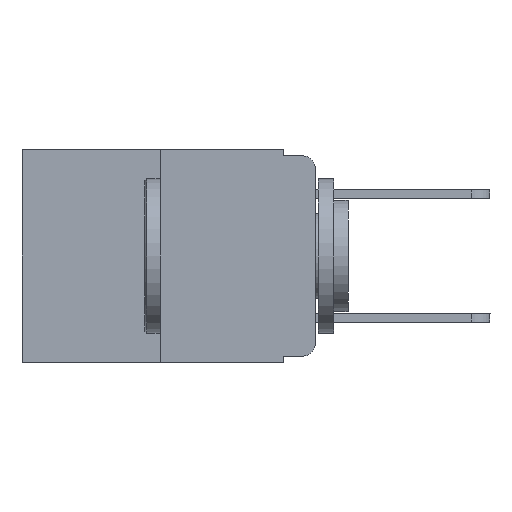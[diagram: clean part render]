
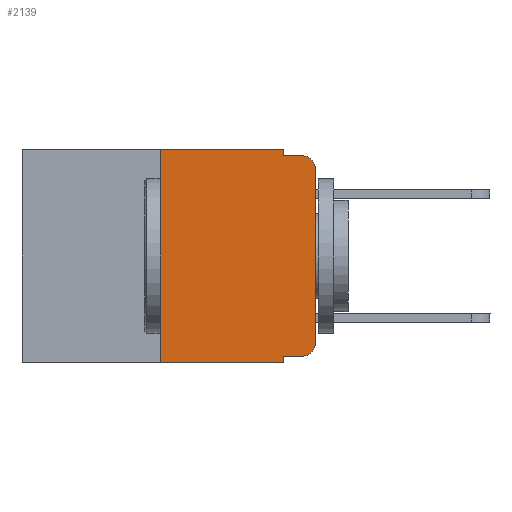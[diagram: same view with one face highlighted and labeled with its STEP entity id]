
A CAD part, left-side view. The second image highlights one B-rep face of the part: STEP entity #2139.
In plain terms, the highlighted planar face has unit normal (-1, 0, 0).
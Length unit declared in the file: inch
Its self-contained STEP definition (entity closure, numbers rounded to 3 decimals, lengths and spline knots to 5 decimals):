
#105 = ORIENTED_EDGE ( 'NONE', *, *, #9672, .T. ) ;
#133 = VERTEX_POINT ( 'NONE', #2165 ) ;
#196 = ORIENTED_EDGE ( 'NONE', *, *, #19127, .T. ) ;
#374 = DIRECTION ( 'NONE',  ( 0., -1., 0. ) ) ;
#551 = CARTESIAN_POINT ( 'NONE',  ( 0., 0.02, -0.333 ) ) ;
#833 = DIRECTION ( 'NONE',  ( 0., -1., 0. ) ) ;
#955 = VECTOR ( 'NONE', #6826, 39.37008 ) ;
#981 = ORIENTED_EDGE ( 'NONE', *, *, #5267, .F. ) ;
#1406 = VECTOR ( 'NONE', #11845, 39.37008 ) ;
#1689 = VECTOR ( 'NONE', #833, 39.37008 ) ;
#2076 = EDGE_CURVE ( 'NONE', #12194, #8898, #11866, .T. ) ;
#2139 = ADVANCED_FACE ( 'NONE', ( #11354 ), #15346, .F. ) ;
#2165 = CARTESIAN_POINT ( 'NONE',  ( 0., 0.02, -0.01 ) ) ;
#2209 = EDGE_CURVE ( 'NONE', #13697, #2356, #12379, .T. ) ;
#2356 = VERTEX_POINT ( 'NONE', #6018 ) ;
#2637 = CARTESIAN_POINT ( 'NONE',  ( 0., 0.25, 0. ) ) ;
#2941 = ORIENTED_EDGE ( 'NONE', *, *, #13623, .T. ) ;
#3417 = CARTESIAN_POINT ( 'NONE',  ( 0., 0.051, -0.01 ) ) ;
#3504 = DIRECTION ( 'NONE',  ( 0., 0., 1. ) ) ;
#3526 = CARTESIAN_POINT ( 'NONE',  ( 0., 0.051, 0. ) ) ;
#3606 = DIRECTION ( 'NONE',  ( 1., 0., 0. ) ) ;
#3746 = CARTESIAN_POINT ( 'NONE',  ( 0., 0.473, 0. ) ) ;
#3792 = ORIENTED_EDGE ( 'NONE', *, *, #3829, .F. ) ;
#3829 = EDGE_CURVE ( 'NONE', #18130, #133, #15954, .T. ) ;
#4917 = LINE ( 'NONE', #19676, #15035 ) ;
#5001 = VECTOR ( 'NONE', #3504, 39.37008 ) ;
#5251 = DIRECTION ( 'NONE',  ( 0., 0., -1. ) ) ;
#5267 = EDGE_CURVE ( 'NONE', #15118, #12194, #14366, .T. ) ;
#5407 = EDGE_LOOP ( 'NONE', ( #14803, #196, #3792, #10433, #10641, #981, #105, #11009, #20525, #2941 ) ) ;
#5794 = DIRECTION ( 'NONE',  ( -1., 0., 0. ) ) ;
#6018 = CARTESIAN_POINT ( 'NONE',  ( 0., 0., -0.03 ) ) ;
#6826 = DIRECTION ( 'NONE',  ( 0., -1., 0. ) ) ;
#7186 = EDGE_CURVE ( 'NONE', #13877, #10578, #13837, .T. ) ;
#7268 = EDGE_CURVE ( 'NONE', #13877, #12577, #12021, .T. ) ;
#7383 = DIRECTION ( 'NONE',  ( 0., 0., 1. ) ) ;
#7666 = CARTESIAN_POINT ( 'NONE',  ( 0., 0.051, 0. ) ) ;
#7942 = VECTOR ( 'NONE', #7383, 39.37008 ) ;
#8195 = CARTESIAN_POINT ( 'NONE',  ( 0., 0., -0.313 ) ) ;
#8267 = CARTESIAN_POINT ( 'NONE',  ( 0., 0.02, -0.313 ) ) ;
#8898 = VERTEX_POINT ( 'NONE', #7666 ) ;
#9183 = LINE ( 'NONE', #14618, #17534 ) ;
#9672 = EDGE_CURVE ( 'NONE', #15118, #10578, #4917, .T. ) ;
#10433 = ORIENTED_EDGE ( 'NONE', *, *, #12267, .F. ) ;
#10578 = VERTEX_POINT ( 'NONE', #10746 ) ;
#10641 = ORIENTED_EDGE ( 'NONE', *, *, #2076, .F. ) ;
#10746 = CARTESIAN_POINT ( 'NONE',  ( 0., 0.051, -0.343 ) ) ;
#11009 = ORIENTED_EDGE ( 'NONE', *, *, #7186, .F. ) ;
#11196 = DIRECTION ( 'NONE',  ( 0., 0., -1. ) ) ;
#11354 = FACE_OUTER_BOUND ( 'NONE', #5407, .T. ) ;
#11516 = AXIS2_PLACEMENT_3D ( 'NONE', #20720, #5794, #13948 ) ;
#11773 = DIRECTION ( 'NONE',  ( 0., -1., 0. ) ) ;
#11845 = DIRECTION ( 'NONE',  ( 0., 0., -1. ) ) ;
#11866 = LINE ( 'NONE', #3746, #955 ) ;
#12021 = LINE ( 'NONE', #15339, #17731 ) ;
#12194 = VERTEX_POINT ( 'NONE', #2637 ) ;
#12210 = CARTESIAN_POINT ( 'NONE',  ( 0., 0., 0. ) ) ;
#12267 = EDGE_CURVE ( 'NONE', #8898, #18130, #9183, .T. ) ;
#12379 = LINE ( 'NONE', #12210, #7942 ) ;
#12577 = VERTEX_POINT ( 'NONE', #551 ) ;
#13520 = CARTESIAN_POINT ( 'NONE',  ( 0., 0.473, 0. ) ) ;
#13589 = CARTESIAN_POINT ( 'NONE',  ( 0., 0.25, -0.343 ) ) ;
#13623 = EDGE_CURVE ( 'NONE', #12577, #13697, #13688, .T. ) ;
#13688 = CIRCLE ( 'NONE', #20913, 0.02 ) ;
#13697 = VERTEX_POINT ( 'NONE', #8195 ) ;
#13837 = LINE ( 'NONE', #3526, #1406 ) ;
#13877 = VERTEX_POINT ( 'NONE', #17135 ) ;
#13948 = DIRECTION ( 'NONE',  ( 0., 0., -1. ) ) ;
#13980 = CARTESIAN_POINT ( 'NONE',  ( 0., 0.051, -0.01 ) ) ;
#14366 = LINE ( 'NONE', #20202, #5001 ) ;
#14618 = CARTESIAN_POINT ( 'NONE',  ( 0., 0.051, 0. ) ) ;
#14803 = ORIENTED_EDGE ( 'NONE', *, *, #2209, .T. ) ;
#15035 = VECTOR ( 'NONE', #11773, 39.37008 ) ;
#15118 = VERTEX_POINT ( 'NONE', #13589 ) ;
#15339 = CARTESIAN_POINT ( 'NONE',  ( 0., 0.051, -0.333 ) ) ;
#15346 = PLANE ( 'NONE',  #16152 ) ;
#15954 = LINE ( 'NONE', #13980, #1689 ) ;
#16152 = AXIS2_PLACEMENT_3D ( 'NONE', #13520, #3606, #5251 ) ;
#17135 = CARTESIAN_POINT ( 'NONE',  ( 0., 0.051, -0.333 ) ) ;
#17534 = VECTOR ( 'NONE', #11196, 39.37008 ) ;
#17731 = VECTOR ( 'NONE', #374, 39.37008 ) ;
#17908 = CIRCLE ( 'NONE', #11516, 0.02 ) ;
#18130 = VERTEX_POINT ( 'NONE', #3417 ) ;
#19127 = EDGE_CURVE ( 'NONE', #2356, #133, #17908, .T. ) ;
#19676 = CARTESIAN_POINT ( 'NONE',  ( 0., 0.473, -0.343 ) ) ;
#20151 = DIRECTION ( 'NONE',  ( 0., 0., -1. ) ) ;
#20158 = DIRECTION ( 'NONE',  ( -1., 0., 0. ) ) ;
#20202 = CARTESIAN_POINT ( 'NONE',  ( 0., 0.25, 0. ) ) ;
#20525 = ORIENTED_EDGE ( 'NONE', *, *, #7268, .T. ) ;
#20720 = CARTESIAN_POINT ( 'NONE',  ( 0., 0.02, -0.03 ) ) ;
#20913 = AXIS2_PLACEMENT_3D ( 'NONE', #8267, #20158, #20151 ) ;
